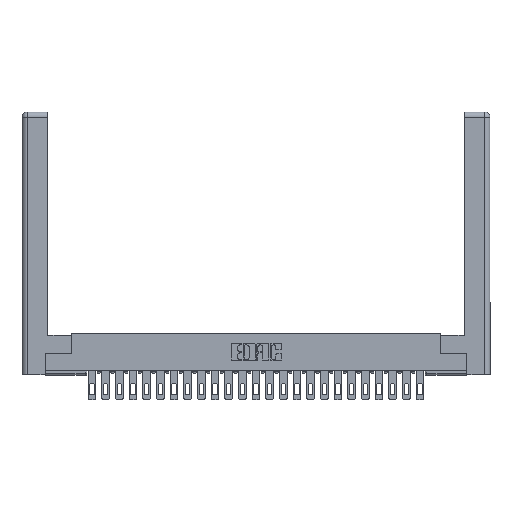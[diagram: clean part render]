
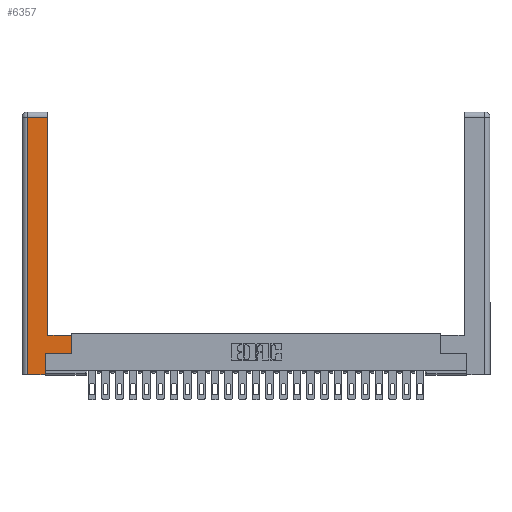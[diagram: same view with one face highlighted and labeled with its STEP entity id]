
A CAD part, top view. The second image highlights one B-rep face of the part: STEP entity #6357.
In plain terms, the highlighted planar face has unit normal (0, 0, 1).
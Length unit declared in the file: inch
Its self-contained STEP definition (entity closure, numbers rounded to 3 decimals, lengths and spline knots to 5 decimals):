
#136 = LINE ( 'NONE', #21975, #1385 ) ;
#353 = CARTESIAN_POINT ( 'NONE',  ( 0.0615, 2.94, 0. ) ) ;
#423 = ORIENTED_EDGE ( 'NONE', *, *, #1782, .T. ) ;
#858 = CARTESIAN_POINT ( 'NONE',  ( 0.295, 3., 0. ) ) ;
#1003 = CARTESIAN_POINT ( 'NONE',  ( 0.265, 0.245, 0. ) ) ;
#1025 = VECTOR ( 'NONE', #1553, 39.37008 ) ;
#1187 = CARTESIAN_POINT ( 'NONE',  ( 0.565, 0.45, 0. ) ) ;
#1385 = VECTOR ( 'NONE', #5653, 39.37008 ) ;
#1432 = DIRECTION ( 'NONE',  ( -1., 0., 0. ) ) ;
#1553 = DIRECTION ( 'NONE',  ( 0., -1., 0. ) ) ;
#1782 = EDGE_CURVE ( 'NONE', #16327, #2209, #25506, .T. ) ;
#1890 = CARTESIAN_POINT ( 'NONE',  ( 0.265, 0.245, 0. ) ) ;
#2209 = VERTEX_POINT ( 'NONE', #21425 ) ;
#2296 = LINE ( 'NONE', #11600, #1025 ) ;
#2634 = DIRECTION ( 'NONE',  ( 0., 1., 0. ) ) ;
#3227 = LINE ( 'NONE', #353, #14204 ) ;
#4322 = LINE ( 'NONE', #1890, #5592 ) ;
#4751 = VERTEX_POINT ( 'NONE', #1003 ) ;
#5076 = CARTESIAN_POINT ( 'NONE',  ( 0.295, 2.94, 0. ) ) ;
#5592 = VECTOR ( 'NONE', #24095, 39.37008 ) ;
#5653 = DIRECTION ( 'NONE',  ( -1., 0., 0. ) ) ;
#5813 = VERTEX_POINT ( 'NONE', #21197 ) ;
#6357 = ADVANCED_FACE ( 'NONE', ( #16206 ), #15112, .F. ) ;
#6618 = VECTOR ( 'NONE', #22882, 39.37008 ) ;
#6697 = VERTEX_POINT ( 'NONE', #1187 ) ;
#8759 = EDGE_CURVE ( 'NONE', #25119, #5813, #3227, .T. ) ;
#8817 = DIRECTION ( 'NONE',  ( -1., 0., 0. ) ) ;
#8927 = ORIENTED_EDGE ( 'NONE', *, *, #12589, .T. ) ;
#9011 = DIRECTION ( 'NONE',  ( 1., 0., 0. ) ) ;
#9145 = CARTESIAN_POINT ( 'NONE',  ( 0.295, 0.45, 0. ) ) ;
#9239 = EDGE_LOOP ( 'NONE', ( #23594, #18792, #25725, #423, #21849, #8927, #15060, #15197 ) ) ;
#9468 = LINE ( 'NONE', #858, #6618 ) ;
#9748 = CARTESIAN_POINT ( 'NONE',  ( 0., 0., 0. ) ) ;
#9936 = EDGE_CURVE ( 'NONE', #11987, #6697, #13499, .T. ) ;
#10489 = EDGE_CURVE ( 'NONE', #2209, #4751, #4322, .T. ) ;
#10696 = AXIS2_PLACEMENT_3D ( 'NONE', #9748, #17582, #1432 ) ;
#11299 = VECTOR ( 'NONE', #25531, 39.37008 ) ;
#11589 = EDGE_CURVE ( 'NONE', #5813, #16327, #2296, .T. ) ;
#11600 = CARTESIAN_POINT ( 'NONE',  ( 0.0615, 0., 0. ) ) ;
#11987 = VERTEX_POINT ( 'NONE', #18654 ) ;
#12589 = EDGE_CURVE ( 'NONE', #4751, #11987, #15142, .T. ) ;
#13423 = CARTESIAN_POINT ( 'NONE',  ( 0.265, 0., 0. ) ) ;
#13499 = LINE ( 'NONE', #20277, #18920 ) ;
#14204 = VECTOR ( 'NONE', #8817, 39.37008 ) ;
#14511 = VECTOR ( 'NONE', #9011, 39.37008 ) ;
#14809 = CARTESIAN_POINT ( 'NONE',  ( 0.565, 0.245, 0. ) ) ;
#14911 = CARTESIAN_POINT ( 'NONE',  ( 0.0615, 0., 0. ) ) ;
#15060 = ORIENTED_EDGE ( 'NONE', *, *, #9936, .T. ) ;
#15112 = PLANE ( 'NONE',  #10696 ) ;
#15142 = LINE ( 'NONE', #14809, #14511 ) ;
#15197 = ORIENTED_EDGE ( 'NONE', *, *, #21531, .T. ) ;
#16206 = FACE_OUTER_BOUND ( 'NONE', #9239, .T. ) ;
#16327 = VERTEX_POINT ( 'NONE', #14911 ) ;
#17582 = DIRECTION ( 'NONE',  ( 0., 0., -1. ) ) ;
#18654 = CARTESIAN_POINT ( 'NONE',  ( 0.565, 0.245, 0. ) ) ;
#18792 = ORIENTED_EDGE ( 'NONE', *, *, #8759, .T. ) ;
#18920 = VECTOR ( 'NONE', #2634, 39.37008 ) ;
#19124 = VERTEX_POINT ( 'NONE', #9145 ) ;
#19128 = EDGE_CURVE ( 'NONE', #19124, #25119, #9468, .T. ) ;
#20277 = CARTESIAN_POINT ( 'NONE',  ( 0.565, 0.45, 0. ) ) ;
#21197 = CARTESIAN_POINT ( 'NONE',  ( 0.0615, 2.94, 0. ) ) ;
#21425 = CARTESIAN_POINT ( 'NONE',  ( 0.265, 0., 0. ) ) ;
#21531 = EDGE_CURVE ( 'NONE', #6697, #19124, #136, .T. ) ;
#21849 = ORIENTED_EDGE ( 'NONE', *, *, #10489, .T. ) ;
#21975 = CARTESIAN_POINT ( 'NONE',  ( 0.295, 0.45, 0. ) ) ;
#22882 = DIRECTION ( 'NONE',  ( 0., 1., 0. ) ) ;
#23594 = ORIENTED_EDGE ( 'NONE', *, *, #19128, .T. ) ;
#24095 = DIRECTION ( 'NONE',  ( 0., 1., 0. ) ) ;
#25119 = VERTEX_POINT ( 'NONE', #5076 ) ;
#25506 = LINE ( 'NONE', #13423, #11299 ) ;
#25531 = DIRECTION ( 'NONE',  ( 1., 0., 0. ) ) ;
#25725 = ORIENTED_EDGE ( 'NONE', *, *, #11589, .T. ) ;
